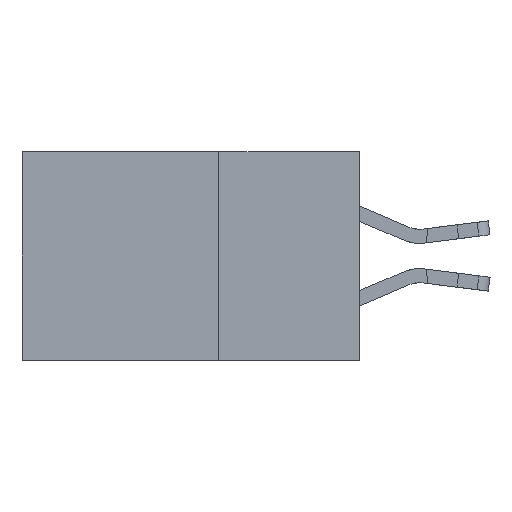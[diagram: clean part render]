
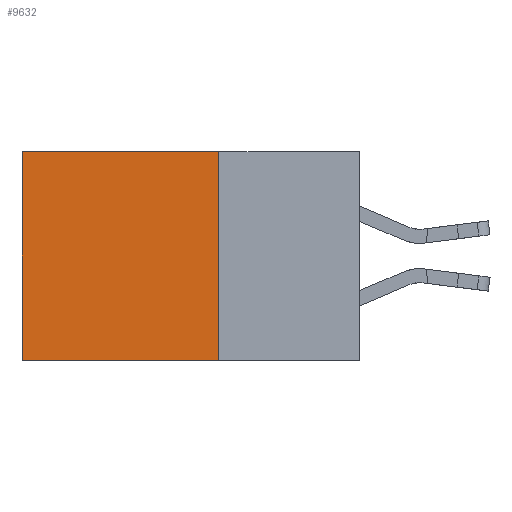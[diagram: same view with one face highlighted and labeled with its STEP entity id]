
A CAD part, left-side view. The second image highlights one B-rep face of the part: STEP entity #9632.
In plain terms, the highlighted planar face has unit normal (-1, 0, 0).
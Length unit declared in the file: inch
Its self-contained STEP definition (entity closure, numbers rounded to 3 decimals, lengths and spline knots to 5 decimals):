
#2 = ORIENTED_EDGE ( 'NONE', *, *, #14615, .F. ) ;
#1050 = EDGE_CURVE ( 'NONE', #11784, #10084, #4209, .T. ) ;
#1110 = CARTESIAN_POINT ( 'NONE',  ( 0.2875, 0.25, 0. ) ) ;
#1332 = CARTESIAN_POINT ( 'NONE',  ( 0.2875, 0.25, 0. ) ) ;
#1656 = DIRECTION ( 'NONE',  ( 0., 0., -1. ) ) ;
#1824 = ORIENTED_EDGE ( 'NONE', *, *, #6359, .T. ) ;
#2463 = EDGE_CURVE ( 'NONE', #11784, #9282, #10449, .T. ) ;
#2960 = LINE ( 'NONE', #13745, #15184 ) ;
#3014 = DIRECTION ( 'NONE',  ( 0., 1., 0. ) ) ;
#4209 = LINE ( 'NONE', #7336, #12205 ) ;
#4291 = CARTESIAN_POINT ( 'NONE',  ( 0.2875, 0.6, 0. ) ) ;
#4624 = ORIENTED_EDGE ( 'NONE', *, *, #2463, .F. ) ;
#5947 = AXIS2_PLACEMENT_3D ( 'NONE', #1110, #13303, #10750 ) ;
#6359 = EDGE_CURVE ( 'NONE', #10084, #14602, #11274, .T. ) ;
#6557 = CARTESIAN_POINT ( 'NONE',  ( 0.2875, 0.6, 0. ) ) ;
#7300 = PLANE ( 'NONE',  #5947 ) ;
#7336 = CARTESIAN_POINT ( 'NONE',  ( 0.2875, 0.25, 0. ) ) ;
#7399 = VECTOR ( 'NONE', #12337, 39.37008 ) ;
#7408 = CARTESIAN_POINT ( 'NONE',  ( 0.2875, 0.25, 0. ) ) ;
#7410 = EDGE_LOOP ( 'NONE', ( #1824, #2, #4624, #13355 ) ) ;
#9049 = CARTESIAN_POINT ( 'NONE',  ( 0.2875, 0.25, -0.37 ) ) ;
#9282 = VERTEX_POINT ( 'NONE', #9049 ) ;
#9632 = ADVANCED_FACE ( 'NONE', ( #11777 ), #7300, .F. ) ;
#10084 = VERTEX_POINT ( 'NONE', #6557 ) ;
#10245 = CARTESIAN_POINT ( 'NONE',  ( 0.2875, 0.6, -0.37 ) ) ;
#10449 = LINE ( 'NONE', #7408, #7399 ) ;
#10750 = DIRECTION ( 'NONE',  ( 0., 0., -1. ) ) ;
#11274 = LINE ( 'NONE', #4291, #14912 ) ;
#11777 = FACE_OUTER_BOUND ( 'NONE', #7410, .T. ) ;
#11784 = VERTEX_POINT ( 'NONE', #1332 ) ;
#12205 = VECTOR ( 'NONE', #13489, 39.37008 ) ;
#12337 = DIRECTION ( 'NONE',  ( 0., 0., -1. ) ) ;
#13303 = DIRECTION ( 'NONE',  ( 1., 0., 0. ) ) ;
#13355 = ORIENTED_EDGE ( 'NONE', *, *, #1050, .T. ) ;
#13489 = DIRECTION ( 'NONE',  ( 0., 1., 0. ) ) ;
#13745 = CARTESIAN_POINT ( 'NONE',  ( 0.2875, 0.25, -0.37 ) ) ;
#14602 = VERTEX_POINT ( 'NONE', #10245 ) ;
#14615 = EDGE_CURVE ( 'NONE', #9282, #14602, #2960, .T. ) ;
#14912 = VECTOR ( 'NONE', #1656, 39.37008 ) ;
#15184 = VECTOR ( 'NONE', #3014, 39.37008 ) ;
